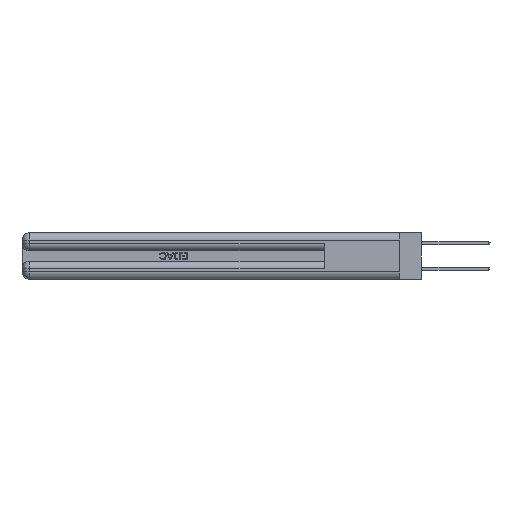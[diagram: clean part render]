
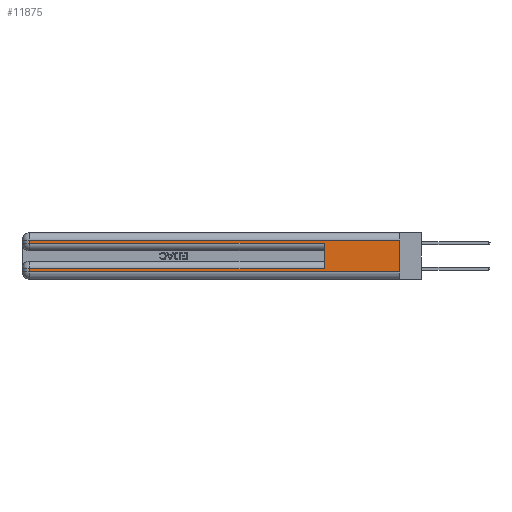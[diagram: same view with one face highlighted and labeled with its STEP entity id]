
A CAD part, left-side view. The second image highlights one B-rep face of the part: STEP entity #11875.
In plain terms, the highlighted planar face has unit normal (-1, 0, 0).
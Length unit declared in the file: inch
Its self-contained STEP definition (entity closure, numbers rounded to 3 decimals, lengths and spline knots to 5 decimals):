
#235 = ORIENTED_EDGE ( 'NONE', *, *, #40265, .F. ) ;
#518 = CARTESIAN_POINT ( 'NONE',  ( 0., 0.6, 0.085 ) ) ;
#1164 = CARTESIAN_POINT ( 'NONE',  ( 0., 2.94, 0.37 ) ) ;
#2252 = CARTESIAN_POINT ( 'NONE',  ( 0., 0., 0.085 ) ) ;
#2834 = VECTOR ( 'NONE', #36491, 39.37008 ) ;
#3430 = VECTOR ( 'NONE', #22563, 39.37008 ) ;
#7394 = DIRECTION ( 'NONE',  ( 0., 0., -1. ) ) ;
#8146 = EDGE_LOOP ( 'NONE', ( #235, #8274, #44031, #30359, #32610, #21983, #10687, #36676 ) ) ;
#8274 = ORIENTED_EDGE ( 'NONE', *, *, #12899, .T. ) ;
#9123 = VERTEX_POINT ( 'NONE', #47732 ) ;
#10254 = VECTOR ( 'NONE', #21816, 39.37008 ) ;
#10687 = ORIENTED_EDGE ( 'NONE', *, *, #16531, .T. ) ;
#11875 = ADVANCED_FACE ( 'NONE', ( #21981 ), #38985, .F. ) ;
#12899 = EDGE_CURVE ( 'NONE', #39970, #39890, #36460, .T. ) ;
#12981 = VECTOR ( 'NONE', #49792, 39.37008 ) ;
#13860 = VERTEX_POINT ( 'NONE', #518 ) ;
#13873 = LINE ( 'NONE', #38015, #3430 ) ;
#14028 = EDGE_CURVE ( 'NONE', #47714, #9123, #42907, .T. ) ;
#14471 = CARTESIAN_POINT ( 'NONE',  ( 0., 0.6, 0.285 ) ) ;
#15290 = VECTOR ( 'NONE', #7394, 39.37008 ) ;
#15976 = DIRECTION ( 'NONE',  ( 0., 0., -1. ) ) ;
#16222 = EDGE_CURVE ( 'NONE', #39890, #33392, #24421, .T. ) ;
#16531 = EDGE_CURVE ( 'NONE', #35478, #47714, #25603, .T. ) ;
#16924 = CARTESIAN_POINT ( 'NONE',  ( 0., 0., 0.31 ) ) ;
#17083 = VECTOR ( 'NONE', #18691, 39.37008 ) ;
#17938 = EDGE_CURVE ( 'NONE', #13860, #35478, #32843, .T. ) ;
#18656 = CARTESIAN_POINT ( 'NONE',  ( 0., 2.94, 0.085 ) ) ;
#18691 = DIRECTION ( 'NONE',  ( 0., 0., -1. ) ) ;
#18853 = CARTESIAN_POINT ( 'NONE',  ( 0., 2.94, 0.06 ) ) ;
#20484 = CARTESIAN_POINT ( 'NONE',  ( 0., 2.94, 0.31 ) ) ;
#20569 = DIRECTION ( 'NONE',  ( 0., 0., -1. ) ) ;
#21816 = DIRECTION ( 'NONE',  ( 0., 1., 0. ) ) ;
#21981 = FACE_OUTER_BOUND ( 'NONE', #8146, .T. ) ;
#21983 = ORIENTED_EDGE ( 'NONE', *, *, #17938, .T. ) ;
#22199 = EDGE_CURVE ( 'NONE', #33392, #22721, #13873, .T. ) ;
#22241 = AXIS2_PLACEMENT_3D ( 'NONE', #35755, #23687, #15976 ) ;
#22563 = DIRECTION ( 'NONE',  ( 0., -1., 0. ) ) ;
#22721 = VERTEX_POINT ( 'NONE', #14471 ) ;
#23687 = DIRECTION ( 'NONE',  ( 1., 0., 0. ) ) ;
#24183 = CARTESIAN_POINT ( 'NONE',  ( 0., 2.94, 0.285 ) ) ;
#24421 = LINE ( 'NONE', #46336, #17083 ) ;
#25264 = EDGE_CURVE ( 'NONE', #13860, #22721, #33756, .T. ) ;
#25603 = LINE ( 'NONE', #1164, #45106 ) ;
#30359 = ORIENTED_EDGE ( 'NONE', *, *, #22199, .T. ) ;
#31804 = LINE ( 'NONE', #42387, #15290 ) ;
#32189 = DIRECTION ( 'NONE',  ( 0., -1., 0. ) ) ;
#32610 = ORIENTED_EDGE ( 'NONE', *, *, #25264, .F. ) ;
#32843 = LINE ( 'NONE', #2252, #10254 ) ;
#33392 = VERTEX_POINT ( 'NONE', #24183 ) ;
#33756 = LINE ( 'NONE', #34081, #12981 ) ;
#34081 = CARTESIAN_POINT ( 'NONE',  ( 0., 0.6, 0.145 ) ) ;
#35478 = VERTEX_POINT ( 'NONE', #18656 ) ;
#35755 = CARTESIAN_POINT ( 'NONE',  ( 0., 0., 0.37 ) ) ;
#36460 = LINE ( 'NONE', #16924, #2834 ) ;
#36491 = DIRECTION ( 'NONE',  ( 0., 1., 0. ) ) ;
#36676 = ORIENTED_EDGE ( 'NONE', *, *, #14028, .T. ) ;
#38015 = CARTESIAN_POINT ( 'NONE',  ( 0., 0., 0.285 ) ) ;
#38985 = PLANE ( 'NONE',  #22241 ) ;
#39890 = VERTEX_POINT ( 'NONE', #20484 ) ;
#39970 = VERTEX_POINT ( 'NONE', #40554 ) ;
#40265 = EDGE_CURVE ( 'NONE', #39970, #9123, #31804, .T. ) ;
#40554 = CARTESIAN_POINT ( 'NONE',  ( 0., 0., 0.31 ) ) ;
#42387 = CARTESIAN_POINT ( 'NONE',  ( 0., 0., 0.37 ) ) ;
#42907 = LINE ( 'NONE', #43433, #44731 ) ;
#43433 = CARTESIAN_POINT ( 'NONE',  ( 0., 0., 0.06 ) ) ;
#44031 = ORIENTED_EDGE ( 'NONE', *, *, #16222, .T. ) ;
#44731 = VECTOR ( 'NONE', #32189, 39.37008 ) ;
#45106 = VECTOR ( 'NONE', #20569, 39.37008 ) ;
#46336 = CARTESIAN_POINT ( 'NONE',  ( 0., 2.94, 0.37 ) ) ;
#47714 = VERTEX_POINT ( 'NONE', #18853 ) ;
#47732 = CARTESIAN_POINT ( 'NONE',  ( 0., 0., 0.06 ) ) ;
#49792 = DIRECTION ( 'NONE',  ( 0., 0., 1. ) ) ;
